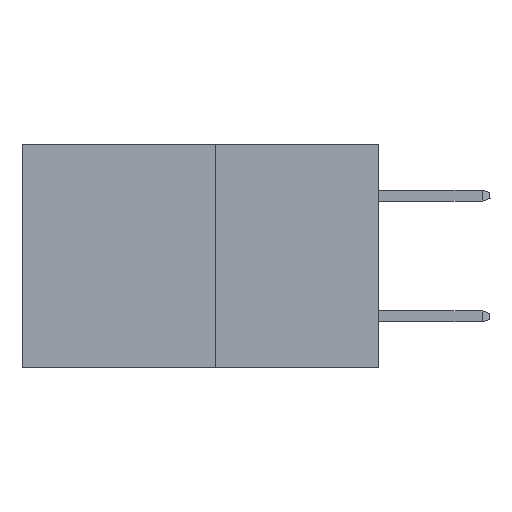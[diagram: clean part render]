
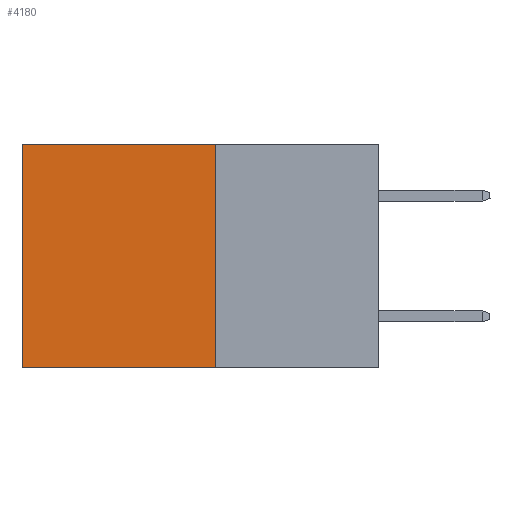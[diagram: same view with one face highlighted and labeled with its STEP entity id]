
A CAD part, left-side view. The second image highlights one B-rep face of the part: STEP entity #4180.
In plain terms, the highlighted planar face has unit normal (-1, 0, 0).
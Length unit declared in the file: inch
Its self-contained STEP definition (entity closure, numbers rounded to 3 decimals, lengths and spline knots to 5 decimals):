
#31 = CARTESIAN_POINT ( 'NONE',  ( 0.277, 0.59, 0. ) ) ;
#144 = LINE ( 'NONE', #13535, #9959 ) ;
#1827 = DIRECTION ( 'NONE',  ( 0., 1., 0. ) ) ;
#2206 = ORIENTED_EDGE ( 'NONE', *, *, #5185, .T. ) ;
#2993 = VERTEX_POINT ( 'NONE', #4253 ) ;
#3532 = LINE ( 'NONE', #16415, #13654 ) ;
#3784 = ORIENTED_EDGE ( 'NONE', *, *, #14000, .F. ) ;
#3797 = VERTEX_POINT ( 'NONE', #9876 ) ;
#4180 = ADVANCED_FACE ( 'NONE', ( #13278 ), #9717, .F. ) ;
#4253 = CARTESIAN_POINT ( 'NONE',  ( 0.277, 0.59, -0.37 ) ) ;
#4292 = DIRECTION ( 'NONE',  ( 0., 1., 0. ) ) ;
#4359 = ORIENTED_EDGE ( 'NONE', *, *, #14295, .T. ) ;
#4982 = CARTESIAN_POINT ( 'NONE',  ( 0.277, 0.27, -0.37 ) ) ;
#5185 = EDGE_CURVE ( 'NONE', #15357, #2993, #3532, .T. ) ;
#5213 = AXIS2_PLACEMENT_3D ( 'NONE', #4982, #12898, #10168 ) ;
#6359 = VECTOR ( 'NONE', #1827, 39.37008 ) ;
#6530 = CARTESIAN_POINT ( 'NONE',  ( 0.277, 0.27, -0.37 ) ) ;
#6695 = VERTEX_POINT ( 'NONE', #10172 ) ;
#7597 = ORIENTED_EDGE ( 'NONE', *, *, #9529, .F. ) ;
#9529 = EDGE_CURVE ( 'NONE', #6695, #2993, #16595, .T. ) ;
#9717 = PLANE ( 'NONE',  #5213 ) ;
#9876 = CARTESIAN_POINT ( 'NONE',  ( 0.277, 0.27, 0. ) ) ;
#9959 = VECTOR ( 'NONE', #4292, 39.37008 ) ;
#10168 = DIRECTION ( 'NONE',  ( 0., 0., -1. ) ) ;
#10172 = CARTESIAN_POINT ( 'NONE',  ( 0.277, 0.27, -0.37 ) ) ;
#10572 = LINE ( 'NONE', #6530, #13939 ) ;
#11180 = EDGE_LOOP ( 'NONE', ( #2206, #7597, #3784, #4359 ) ) ;
#12898 = DIRECTION ( 'NONE',  ( 1., 0., 0. ) ) ;
#13278 = FACE_OUTER_BOUND ( 'NONE', #11180, .T. ) ;
#13535 = CARTESIAN_POINT ( 'NONE',  ( 0.277, 0.27, 0. ) ) ;
#13593 = CARTESIAN_POINT ( 'NONE',  ( 0.277, 0.27, -0.37 ) ) ;
#13654 = VECTOR ( 'NONE', #14133, 39.37008 ) ;
#13939 = VECTOR ( 'NONE', #15568, 39.37008 ) ;
#14000 = EDGE_CURVE ( 'NONE', #3797, #6695, #10572, .T. ) ;
#14133 = DIRECTION ( 'NONE',  ( 0., 0., -1. ) ) ;
#14295 = EDGE_CURVE ( 'NONE', #3797, #15357, #144, .T. ) ;
#15357 = VERTEX_POINT ( 'NONE', #31 ) ;
#15568 = DIRECTION ( 'NONE',  ( 0., 0., -1. ) ) ;
#16415 = CARTESIAN_POINT ( 'NONE',  ( 0.277, 0.59, -0.37 ) ) ;
#16595 = LINE ( 'NONE', #13593, #6359 ) ;
